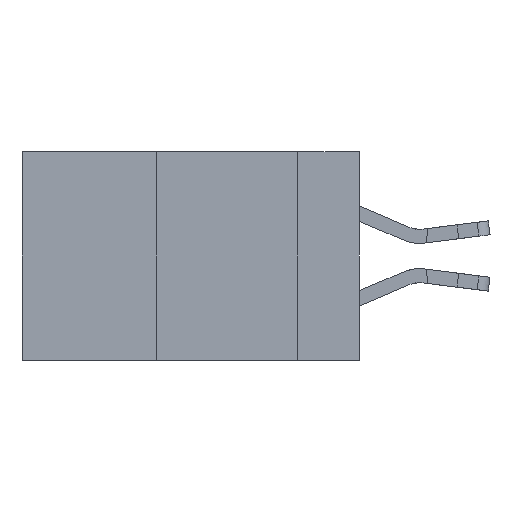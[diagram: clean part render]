
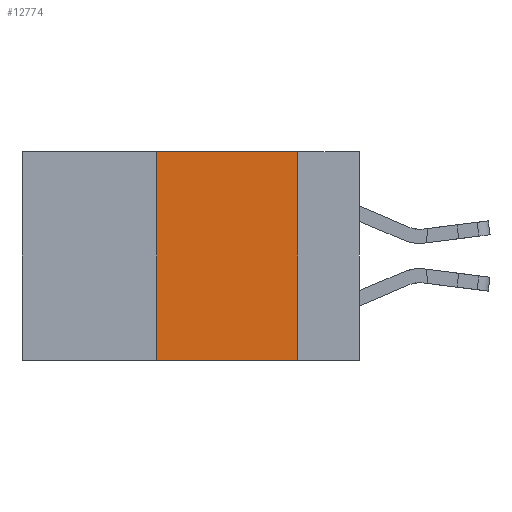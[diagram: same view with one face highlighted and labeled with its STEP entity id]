
A CAD part, left-side view. The second image highlights one B-rep face of the part: STEP entity #12774.
In plain terms, the highlighted planar face has unit normal (-1, 0, 0).
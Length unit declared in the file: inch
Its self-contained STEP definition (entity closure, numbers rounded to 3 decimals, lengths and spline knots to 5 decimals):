
#290 = VERTEX_POINT ( 'NONE', #8304 ) ;
#419 = EDGE_CURVE ( 'NONE', #16708, #8908, #979, .T. ) ;
#979 = LINE ( 'NONE', #5326, #5463 ) ;
#1441 = CARTESIAN_POINT ( 'NONE',  ( 0., 0.11, -0.37 ) ) ;
#1544 = ORIENTED_EDGE ( 'NONE', *, *, #16380, .F. ) ;
#2104 = LINE ( 'NONE', #15262, #18753 ) ;
#2325 = DIRECTION ( 'NONE',  ( 0., 0., -1. ) ) ;
#2614 = FACE_OUTER_BOUND ( 'NONE', #5726, .T. ) ;
#3819 = DIRECTION ( 'NONE',  ( 1., 0., 0. ) ) ;
#4881 = ORIENTED_EDGE ( 'NONE', *, *, #11262, .T. ) ;
#5326 = CARTESIAN_POINT ( 'NONE',  ( 0., 0.36, 0. ) ) ;
#5463 = VECTOR ( 'NONE', #18988, 39.37008 ) ;
#5726 = EDGE_LOOP ( 'NONE', ( #1544, #16348, #5956, #4881 ) ) ;
#5956 = ORIENTED_EDGE ( 'NONE', *, *, #419, .F. ) ;
#6132 = AXIS2_PLACEMENT_3D ( 'NONE', #16171, #3819, #2325 ) ;
#6254 = DIRECTION ( 'NONE',  ( 0., -1., 0. ) ) ;
#6815 = DIRECTION ( 'NONE',  ( 0., 0., -1. ) ) ;
#7284 = DIRECTION ( 'NONE',  ( 0., -1., 0. ) ) ;
#8304 = CARTESIAN_POINT ( 'NONE',  ( 0., 0.11, 0. ) ) ;
#8908 = VERTEX_POINT ( 'NONE', #16005 ) ;
#11262 = EDGE_CURVE ( 'NONE', #16708, #18517, #13691, .T. ) ;
#11798 = EDGE_CURVE ( 'NONE', #8908, #290, #2104, .T. ) ;
#12774 = ADVANCED_FACE ( 'NONE', ( #2614 ), #17749, .F. ) ;
#13691 = LINE ( 'NONE', #17864, #18472 ) ;
#15262 = CARTESIAN_POINT ( 'NONE',  ( 0., 0.6, 0. ) ) ;
#15625 = LINE ( 'NONE', #18882, #17602 ) ;
#16005 = CARTESIAN_POINT ( 'NONE',  ( 0., 0.36, 0. ) ) ;
#16171 = CARTESIAN_POINT ( 'NONE',  ( 0., 0.6, 0. ) ) ;
#16348 = ORIENTED_EDGE ( 'NONE', *, *, #11798, .F. ) ;
#16380 = EDGE_CURVE ( 'NONE', #290, #18517, #15625, .T. ) ;
#16595 = CARTESIAN_POINT ( 'NONE',  ( 0., 0.36, -0.37 ) ) ;
#16708 = VERTEX_POINT ( 'NONE', #16595 ) ;
#17602 = VECTOR ( 'NONE', #6815, 39.37008 ) ;
#17749 = PLANE ( 'NONE',  #6132 ) ;
#17864 = CARTESIAN_POINT ( 'NONE',  ( 0., 0.6, -0.37 ) ) ;
#18472 = VECTOR ( 'NONE', #7284, 39.37008 ) ;
#18517 = VERTEX_POINT ( 'NONE', #1441 ) ;
#18753 = VECTOR ( 'NONE', #6254, 39.37008 ) ;
#18882 = CARTESIAN_POINT ( 'NONE',  ( 0., 0.11, 0. ) ) ;
#18988 = DIRECTION ( 'NONE',  ( 0., 0., 1. ) ) ;
